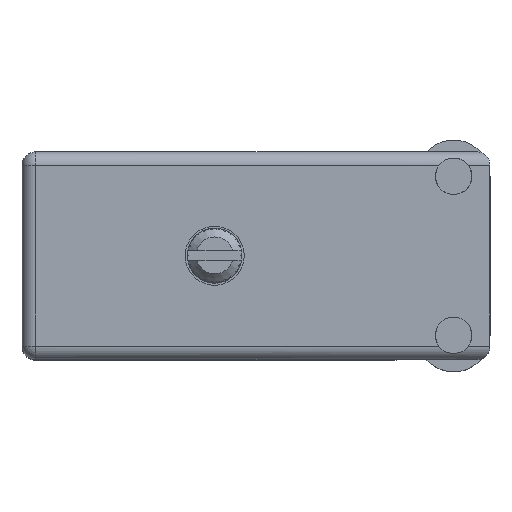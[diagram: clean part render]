
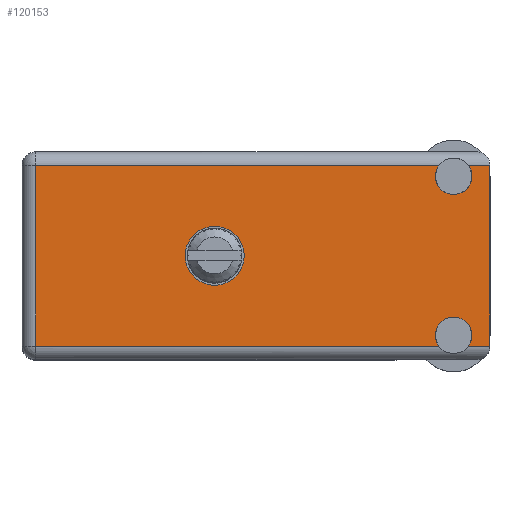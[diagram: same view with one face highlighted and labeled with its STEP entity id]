
A CAD part, top view. The second image highlights one B-rep face of the part: STEP entity #120153.
In plain terms, the highlighted face is planar.
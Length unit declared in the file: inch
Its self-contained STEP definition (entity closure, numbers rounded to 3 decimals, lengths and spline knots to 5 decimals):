
#48 = EDGE_LOOP ( 'NONE', ( #69819, #107584 ) ) ;
#1590 = EDGE_CURVE ( 'NONE', #108651, #108469, #52067, .T. ) ;
#2174 = VERTEX_POINT ( 'NONE', #30836 ) ;
#3087 = DIRECTION ( 'NONE',  ( -1., 0., 0. ) ) ;
#3261 = PLANE ( 'NONE',  #146940 ) ;
#4918 = VERTEX_POINT ( 'NONE', #36694 ) ;
#6137 = CARTESIAN_POINT ( 'NONE',  ( 0.047, 0.906, -0.047 ) ) ;
#6642 = DIRECTION ( 'NONE',  ( 1., 0., 0. ) ) ;
#7698 = CARTESIAN_POINT ( 'NONE',  ( 1.484, 0.906, -0.631 ) ) ;
#12604 = DIRECTION ( 'NONE',  ( 0., 0., 1. ) ) ;
#12779 = VECTOR ( 'NONE', #6642, 39.37008 ) ;
#15466 = ORIENTED_EDGE ( 'NONE', *, *, #71255, .F. ) ;
#19852 = VERTEX_POINT ( 'NONE', #33626 ) ;
#21145 = FACE_OUTER_BOUND ( 'NONE', #63168, .T. ) ;
#21872 = CARTESIAN_POINT ( 'NONE',  ( 1.609, 0.906, -0.668 ) ) ;
#24995 = CIRCLE ( 'NONE', #171834, 0.0625 ) ;
#26148 = ORIENTED_EDGE ( 'NONE', *, *, #170499, .F. ) ;
#29499 = DIRECTION ( 'NONE',  ( 1., 0., 0. ) ) ;
#30486 = LINE ( 'NONE', #108079, #12779 ) ;
#30803 = CARTESIAN_POINT ( 'NONE',  ( 0., 0.906, -0.715 ) ) ;
#30836 = CARTESIAN_POINT ( 'NONE',  ( 0.047, 0.906, -0.668 ) ) ;
#32487 = CARTESIAN_POINT ( 'NONE',  ( 0., 0.906, -0.668 ) ) ;
#32789 = LINE ( 'NONE', #32487, #113533 ) ;
#32998 = CARTESIAN_POINT ( 'NONE',  ( 1.484, 0.906, -0.1465 ) ) ;
#33626 = CARTESIAN_POINT ( 'NONE',  ( 0.6625, 0.906, -0.256 ) ) ;
#35862 = DIRECTION ( 'NONE',  ( 0., 1., 0. ) ) ;
#36694 = CARTESIAN_POINT ( 'NONE',  ( 1.43363, 0.906, -0.047 ) ) ;
#37100 = EDGE_CURVE ( 'NONE', #56489, #4918, #126822, .T. ) ;
#38646 = DIRECTION ( 'NONE',  ( 0., 0., 1. ) ) ;
#39830 = CIRCLE ( 'NONE', #128178, 0.1015 ) ;
#43736 = DIRECTION ( 'NONE',  ( 0., 1., 0. ) ) ;
#46168 = ORIENTED_EDGE ( 'NONE', *, *, #128743, .F. ) ;
#48476 = VECTOR ( 'NONE', #29499, 39.37008 ) ;
#49955 = CARTESIAN_POINT ( 'NONE',  ( 1.53437, 0.906, -0.047 ) ) ;
#51579 = DIRECTION ( 'NONE',  ( -1., 0., 0. ) ) ;
#52027 = DIRECTION ( 'NONE',  ( 0., 0., 1. ) ) ;
#52067 = LINE ( 'NONE', #180069, #168777 ) ;
#52714 = DIRECTION ( 'NONE',  ( 0., 0., 1. ) ) ;
#53101 = CARTESIAN_POINT ( 'NONE',  ( 1.484, 0.906, -0.084 ) ) ;
#53343 = CARTESIAN_POINT ( 'NONE',  ( 0.047, 0.906, -0.715 ) ) ;
#54036 = EDGE_CURVE ( 'NONE', #108005, #19852, #39830, .T. ) ;
#56489 = VERTEX_POINT ( 'NONE', #32998 ) ;
#57635 = CARTESIAN_POINT ( 'NONE',  ( 1.609, 0.906, -0.047 ) ) ;
#61673 = EDGE_CURVE ( 'NONE', #19852, #108005, #152777, .T. ) ;
#61956 = LINE ( 'NONE', #57635, #48476 ) ;
#63168 = EDGE_LOOP ( 'NONE', ( #170874, #155041, #46168, #181146, #98802, #166353, #15466, #26148, #93463, #70218 ) ) ;
#63701 = VECTOR ( 'NONE', #38646, 39.37008 ) ;
#66779 = CARTESIAN_POINT ( 'NONE',  ( 1.609, 0.906, 0. ) ) ;
#69513 = CARTESIAN_POINT ( 'NONE',  ( 1.484, 0.906, -0.631 ) ) ;
#69819 = ORIENTED_EDGE ( 'NONE', *, *, #61673, .F. ) ;
#70218 = ORIENTED_EDGE ( 'NONE', *, *, #146913, .T. ) ;
#71255 = EDGE_CURVE ( 'NONE', #117610, #108469, #175220, .T. ) ;
#73984 = CARTESIAN_POINT ( 'NONE',  ( 1.43363, 0.906, -0.668 ) ) ;
#77285 = AXIS2_PLACEMENT_3D ( 'NONE', #115776, #127054, #185397 ) ;
#84546 = EDGE_CURVE ( 'NONE', #94420, #88401, #30486, .T. ) ;
#88401 = VERTEX_POINT ( 'NONE', #181231 ) ;
#88946 = VERTEX_POINT ( 'NONE', #6137 ) ;
#93463 = ORIENTED_EDGE ( 'NONE', *, *, #99467, .T. ) ;
#94420 = VERTEX_POINT ( 'NONE', #49955 ) ;
#96450 = EDGE_CURVE ( 'NONE', #108651, #88401, #151051, .T. ) ;
#96941 = DIRECTION ( 'NONE',  ( 0., 0., 1. ) ) ;
#98802 = ORIENTED_EDGE ( 'NONE', *, *, #96450, .F. ) ;
#99467 = EDGE_CURVE ( 'NONE', #145672, #2174, #32789, .T. ) ;
#102734 = AXIS2_PLACEMENT_3D ( 'NONE', #137229, #107249, #52027 ) ;
#103176 = CARTESIAN_POINT ( 'NONE',  ( 0.6625, 0.906, -0.3575 ) ) ;
#107249 = DIRECTION ( 'NONE',  ( 0., 1., 0. ) ) ;
#107584 = ORIENTED_EDGE ( 'NONE', *, *, #54036, .F. ) ;
#108005 = VERTEX_POINT ( 'NONE', #130447 ) ;
#108079 = CARTESIAN_POINT ( 'NONE',  ( 1.609, 0.906, -0.047 ) ) ;
#108469 = VERTEX_POINT ( 'NONE', #185625 ) ;
#108486 = AXIS2_PLACEMENT_3D ( 'NONE', #53101, #182845, #96941 ) ;
#108651 = VERTEX_POINT ( 'NONE', #21872 ) ;
#113533 = VECTOR ( 'NONE', #3087, 39.37008 ) ;
#115776 = CARTESIAN_POINT ( 'NONE',  ( 1.484, 0.906, -0.084 ) ) ;
#117610 = VERTEX_POINT ( 'NONE', #136235 ) ;
#120153 = ADVANCED_FACE ( 'NONE', ( #169129, #21145 ), #3261, .T. ) ;
#126822 = CIRCLE ( 'NONE', #77285, 0.0625 ) ;
#127054 = DIRECTION ( 'NONE',  ( 0., 1., 0. ) ) ;
#128178 = AXIS2_PLACEMENT_3D ( 'NONE', #103176, #43736, #143917 ) ;
#128743 = EDGE_CURVE ( 'NONE', #94420, #56489, #169932, .T. ) ;
#130447 = CARTESIAN_POINT ( 'NONE',  ( 0.6625, 0.906, -0.459 ) ) ;
#136235 = CARTESIAN_POINT ( 'NONE',  ( 1.484, 0.906, -0.5685 ) ) ;
#137229 = CARTESIAN_POINT ( 'NONE',  ( 0.6625, 0.906, -0.3575 ) ) ;
#140865 = LINE ( 'NONE', #53343, #147481 ) ;
#143917 = DIRECTION ( 'NONE',  ( 0., 0., 1. ) ) ;
#145672 = VERTEX_POINT ( 'NONE', #73984 ) ;
#146913 = EDGE_CURVE ( 'NONE', #2174, #88946, #140865, .T. ) ;
#146940 = AXIS2_PLACEMENT_3D ( 'NONE', #30803, #173631, #147259 ) ;
#147259 = DIRECTION ( 'NONE',  ( 0., 0., 1. ) ) ;
#147481 = VECTOR ( 'NONE', #52714, 39.37008 ) ;
#151051 = LINE ( 'NONE', #66779, #63701 ) ;
#152380 = AXIS2_PLACEMENT_3D ( 'NONE', #7698, #35862, #179333 ) ;
#152777 = CIRCLE ( 'NONE', #102734, 0.1015 ) ;
#155041 = ORIENTED_EDGE ( 'NONE', *, *, #37100, .F. ) ;
#161837 = EDGE_CURVE ( 'NONE', #88946, #4918, #61956, .T. ) ;
#166353 = ORIENTED_EDGE ( 'NONE', *, *, #1590, .T. ) ;
#168777 = VECTOR ( 'NONE', #51579, 39.37008 ) ;
#169129 = FACE_BOUND ( 'NONE', #48, .T. ) ;
#169793 = DIRECTION ( 'NONE',  ( 0., 1., 0. ) ) ;
#169932 = CIRCLE ( 'NONE', #108486, 0.0625 ) ;
#170499 = EDGE_CURVE ( 'NONE', #145672, #117610, #24995, .T. ) ;
#170874 = ORIENTED_EDGE ( 'NONE', *, *, #161837, .T. ) ;
#171834 = AXIS2_PLACEMENT_3D ( 'NONE', #69513, #169793, #12604 ) ;
#173631 = DIRECTION ( 'NONE',  ( 0., 1., 0. ) ) ;
#175220 = CIRCLE ( 'NONE', #152380, 0.0625 ) ;
#179333 = DIRECTION ( 'NONE',  ( 0., 0., 1. ) ) ;
#180069 = CARTESIAN_POINT ( 'NONE',  ( 0., 0.906, -0.668 ) ) ;
#181146 = ORIENTED_EDGE ( 'NONE', *, *, #84546, .T. ) ;
#181231 = CARTESIAN_POINT ( 'NONE',  ( 1.609, 0.906, -0.047 ) ) ;
#182845 = DIRECTION ( 'NONE',  ( 0., 1., 0. ) ) ;
#185397 = DIRECTION ( 'NONE',  ( 0., 0., 1. ) ) ;
#185625 = CARTESIAN_POINT ( 'NONE',  ( 1.53437, 0.906, -0.668 ) ) ;
